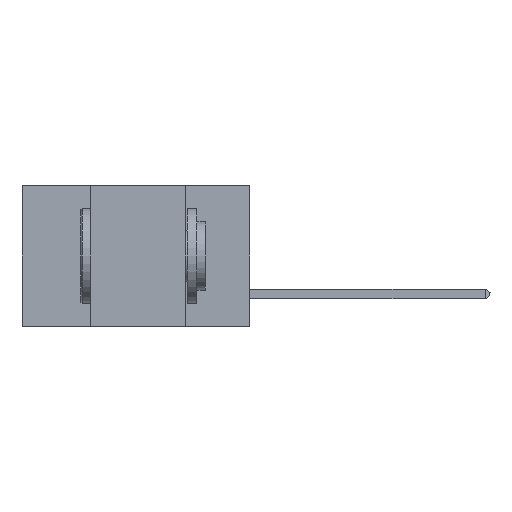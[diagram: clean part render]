
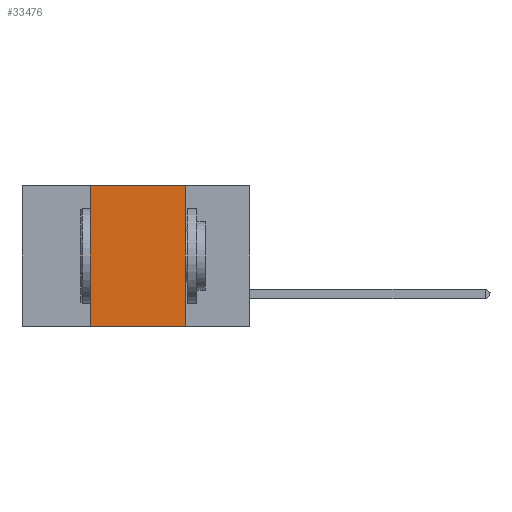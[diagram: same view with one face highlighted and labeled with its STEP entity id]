
A CAD part, left-side view. The second image highlights one B-rep face of the part: STEP entity #33476.
In plain terms, the highlighted planar face has unit normal (-1, 0, 0).
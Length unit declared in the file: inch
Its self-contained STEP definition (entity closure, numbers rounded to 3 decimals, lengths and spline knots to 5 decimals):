
#4449 = ORIENTED_EDGE ( 'NONE', *, *, #46140, .F. ) ;
#4995 = VERTEX_POINT ( 'NONE', #9785 ) ;
#6348 = CARTESIAN_POINT ( 'NONE',  ( 0., 0.6, 0. ) ) ;
#6974 = FACE_OUTER_BOUND ( 'NONE', #12960, .T. ) ;
#8970 = DIRECTION ( 'NONE',  ( 0., 0., -1. ) ) ;
#9206 = DIRECTION ( 'NONE',  ( 0., 0., -1. ) ) ;
#9397 = VECTOR ( 'NONE', #8970, 39.37008 ) ;
#9785 = CARTESIAN_POINT ( 'NONE',  ( 0., 0.17, -0.37 ) ) ;
#10804 = ORIENTED_EDGE ( 'NONE', *, *, #24274, .F. ) ;
#11472 = VECTOR ( 'NONE', #42875, 39.37008 ) ;
#11759 = EDGE_CURVE ( 'NONE', #22573, #4995, #34150, .T. ) ;
#12960 = EDGE_LOOP ( 'NONE', ( #10804, #14518, #4449, #21250 ) ) ;
#13200 = AXIS2_PLACEMENT_3D ( 'NONE', #39822, #43891, #9206 ) ;
#14518 = ORIENTED_EDGE ( 'NONE', *, *, #17182, .F. ) ;
#17182 = EDGE_CURVE ( 'NONE', #43293, #34244, #25338, .T. ) ;
#19476 = CARTESIAN_POINT ( 'NONE',  ( 0., 0.17, 0. ) ) ;
#19738 = LINE ( 'NONE', #44709, #9397 ) ;
#21250 = ORIENTED_EDGE ( 'NONE', *, *, #11759, .T. ) ;
#22573 = VERTEX_POINT ( 'NONE', #49611 ) ;
#23701 = VECTOR ( 'NONE', #29142, 39.37008 ) ;
#24274 = EDGE_CURVE ( 'NONE', #34244, #4995, #19738, .T. ) ;
#24685 = CARTESIAN_POINT ( 'NONE',  ( 0., 0.42, 0. ) ) ;
#25338 = LINE ( 'NONE', #6348, #30290 ) ;
#29142 = DIRECTION ( 'NONE',  ( 0., -1., 0. ) ) ;
#30290 = VECTOR ( 'NONE', #33532, 39.37008 ) ;
#33476 = ADVANCED_FACE ( 'NONE', ( #6974 ), #39647, .F. ) ;
#33532 = DIRECTION ( 'NONE',  ( 0., -1., 0. ) ) ;
#34150 = LINE ( 'NONE', #45184, #23701 ) ;
#34244 = VERTEX_POINT ( 'NONE', #19476 ) ;
#34575 = CARTESIAN_POINT ( 'NONE',  ( 0., 0.42, 0. ) ) ;
#39647 = PLANE ( 'NONE',  #13200 ) ;
#39822 = CARTESIAN_POINT ( 'NONE',  ( 0., 0.6, 0. ) ) ;
#42875 = DIRECTION ( 'NONE',  ( 0., 0., 1. ) ) ;
#43293 = VERTEX_POINT ( 'NONE', #24685 ) ;
#43891 = DIRECTION ( 'NONE',  ( 1., 0., 0. ) ) ;
#44325 = LINE ( 'NONE', #34575, #11472 ) ;
#44709 = CARTESIAN_POINT ( 'NONE',  ( 0., 0.17, 0. ) ) ;
#45184 = CARTESIAN_POINT ( 'NONE',  ( 0., 0.6, -0.37 ) ) ;
#46140 = EDGE_CURVE ( 'NONE', #22573, #43293, #44325, .T. ) ;
#49611 = CARTESIAN_POINT ( 'NONE',  ( 0., 0.42, -0.37 ) ) ;
